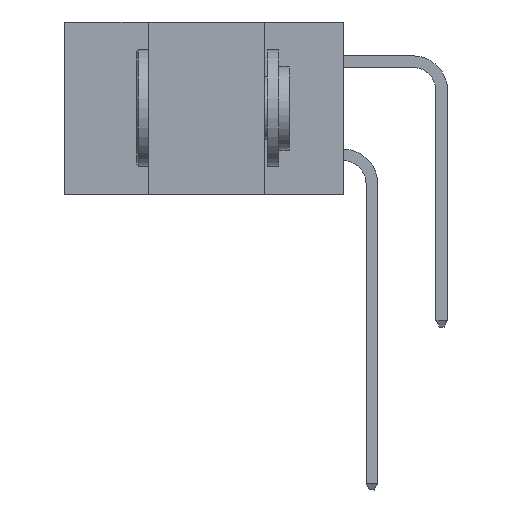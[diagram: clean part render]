
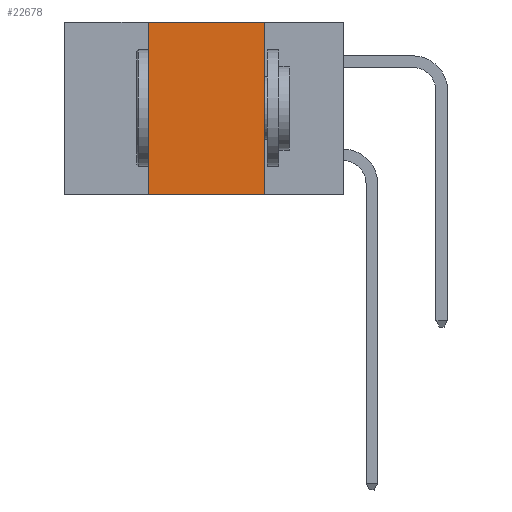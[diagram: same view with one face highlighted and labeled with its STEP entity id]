
A CAD part, left-side view. The second image highlights one B-rep face of the part: STEP entity #22678.
In plain terms, the highlighted planar face has unit normal (-1, 0, 0).
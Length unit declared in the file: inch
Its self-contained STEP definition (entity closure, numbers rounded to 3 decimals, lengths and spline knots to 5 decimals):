
#41 = CARTESIAN_POINT ( 'NONE',  ( 0., 0.42, -0.37 ) ) ;
#183 = ORIENTED_EDGE ( 'NONE', *, *, #28532, .F. ) ;
#397 = VECTOR ( 'NONE', #17964, 39.37008 ) ;
#1464 = VECTOR ( 'NONE', #23425, 39.37008 ) ;
#2035 = EDGE_CURVE ( 'NONE', #14551, #19014, #2463, .T. ) ;
#2463 = LINE ( 'NONE', #25102, #13561 ) ;
#4140 = AXIS2_PLACEMENT_3D ( 'NONE', #18675, #15731, #13487 ) ;
#4539 = DIRECTION ( 'NONE',  ( 0., 0., 1. ) ) ;
#8721 = ORIENTED_EDGE ( 'NONE', *, *, #29338, .F. ) ;
#8862 = EDGE_CURVE ( 'NONE', #14551, #21757, #20208, .T. ) ;
#8946 = CARTESIAN_POINT ( 'NONE',  ( 0., 0.6, -0.37 ) ) ;
#8948 = DIRECTION ( 'NONE',  ( 0., 0., -1. ) ) ;
#12034 = CARTESIAN_POINT ( 'NONE',  ( 0., 0.42, 0. ) ) ;
#12100 = EDGE_LOOP ( 'NONE', ( #183, #8721, #15349, #24606 ) ) ;
#12774 = CARTESIAN_POINT ( 'NONE',  ( 0., 0.17, 0. ) ) ;
#13487 = DIRECTION ( 'NONE',  ( 0., 0., -1. ) ) ;
#13561 = VECTOR ( 'NONE', #4539, 39.37008 ) ;
#14551 = VERTEX_POINT ( 'NONE', #41 ) ;
#15349 = ORIENTED_EDGE ( 'NONE', *, *, #2035, .F. ) ;
#15578 = PLANE ( 'NONE',  #4140 ) ;
#15731 = DIRECTION ( 'NONE',  ( 1., 0., 0. ) ) ;
#16270 = FACE_OUTER_BOUND ( 'NONE', #12100, .T. ) ;
#17964 = DIRECTION ( 'NONE',  ( 0., -1., 0. ) ) ;
#18675 = CARTESIAN_POINT ( 'NONE',  ( 0., 0.6, 0. ) ) ;
#19014 = VERTEX_POINT ( 'NONE', #12034 ) ;
#20208 = LINE ( 'NONE', #8946, #397 ) ;
#20743 = CARTESIAN_POINT ( 'NONE',  ( 0., 0.17, -0.37 ) ) ;
#21757 = VERTEX_POINT ( 'NONE', #20743 ) ;
#22604 = LINE ( 'NONE', #26968, #27754 ) ;
#22678 = ADVANCED_FACE ( 'NONE', ( #16270 ), #15578, .F. ) ;
#23279 = LINE ( 'NONE', #26542, #1464 ) ;
#23425 = DIRECTION ( 'NONE',  ( 0., -1., 0. ) ) ;
#23493 = VERTEX_POINT ( 'NONE', #12774 ) ;
#24606 = ORIENTED_EDGE ( 'NONE', *, *, #8862, .T. ) ;
#25102 = CARTESIAN_POINT ( 'NONE',  ( 0., 0.42, -0.37 ) ) ;
#26542 = CARTESIAN_POINT ( 'NONE',  ( 0., 0.6, 0. ) ) ;
#26968 = CARTESIAN_POINT ( 'NONE',  ( 0., 0.17, -0.37 ) ) ;
#27754 = VECTOR ( 'NONE', #8948, 39.37008 ) ;
#28532 = EDGE_CURVE ( 'NONE', #23493, #21757, #22604, .T. ) ;
#29338 = EDGE_CURVE ( 'NONE', #19014, #23493, #23279, .T. ) ;
